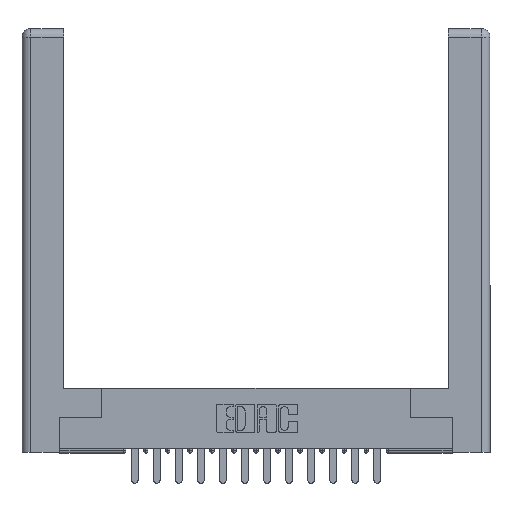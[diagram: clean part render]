
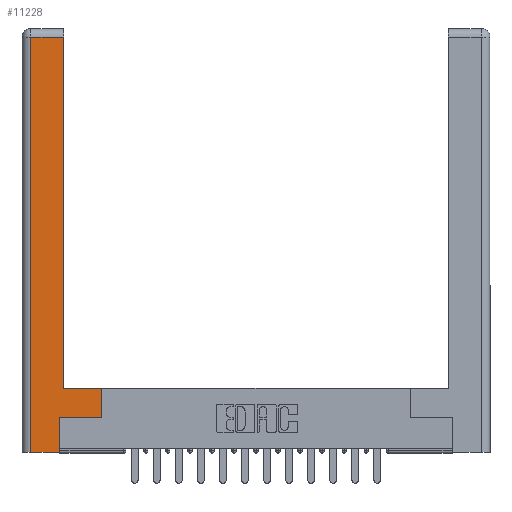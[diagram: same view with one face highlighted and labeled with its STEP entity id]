
A CAD part, top view. The second image highlights one B-rep face of the part: STEP entity #11228.
In plain terms, the highlighted planar face has unit normal (0, 0, 1).
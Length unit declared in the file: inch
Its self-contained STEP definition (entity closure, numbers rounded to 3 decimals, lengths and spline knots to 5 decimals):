
#159 = VECTOR ( 'NONE', #10694, 39.37008 ) ;
#161 = CARTESIAN_POINT ( 'NONE',  ( 0.565, 0.245, 0. ) ) ;
#164 = ORIENTED_EDGE ( 'NONE', *, *, #7320, .T. ) ;
#1499 = EDGE_CURVE ( 'NONE', #12474, #10708, #16077, .T. ) ;
#1503 = EDGE_CURVE ( 'NONE', #18633, #8647, #7940, .T. ) ;
#1504 = DIRECTION ( 'NONE',  ( 1., 0., 0. ) ) ;
#1714 = CARTESIAN_POINT ( 'NONE',  ( 0.295, 3., 0. ) ) ;
#1755 = DIRECTION ( 'NONE',  ( 0., -1., 0. ) ) ;
#2176 = VECTOR ( 'NONE', #12103, 39.37008 ) ;
#2252 = AXIS2_PLACEMENT_3D ( 'NONE', #10477, #3153, #14984 ) ;
#2277 = VECTOR ( 'NONE', #12671, 39.37008 ) ;
#2323 = CARTESIAN_POINT ( 'NONE',  ( 0.295, 2.94, 0. ) ) ;
#2669 = ORIENTED_EDGE ( 'NONE', *, *, #18266, .T. ) ;
#2887 = VECTOR ( 'NONE', #1504, 39.37008 ) ;
#3153 = DIRECTION ( 'NONE',  ( 0., 0., -1. ) ) ;
#3246 = CARTESIAN_POINT ( 'NONE',  ( 0.265, 0.245, 0. ) ) ;
#3468 = EDGE_LOOP ( 'NONE', ( #6511, #2669, #12548, #16633, #18018, #6782, #164, #15457 ) ) ;
#4203 = FACE_OUTER_BOUND ( 'NONE', #3468, .T. ) ;
#4240 = VECTOR ( 'NONE', #1755, 39.37008 ) ;
#5693 = CARTESIAN_POINT ( 'NONE',  ( 0.0615, 2.94, 0. ) ) ;
#6391 = EDGE_CURVE ( 'NONE', #10708, #11615, #10621, .T. ) ;
#6511 = ORIENTED_EDGE ( 'NONE', *, *, #16012, .T. ) ;
#6564 = DIRECTION ( 'NONE',  ( 0., 1., 0. ) ) ;
#6698 = VECTOR ( 'NONE', #16468, 39.37008 ) ;
#6782 = ORIENTED_EDGE ( 'NONE', *, *, #1503, .T. ) ;
#7222 = DIRECTION ( 'NONE',  ( 1., 0., 0. ) ) ;
#7320 = EDGE_CURVE ( 'NONE', #8647, #16659, #12195, .T. ) ;
#7625 = CARTESIAN_POINT ( 'NONE',  ( 0.565, 0.45, 0. ) ) ;
#7712 = VERTEX_POINT ( 'NONE', #18639 ) ;
#7940 = LINE ( 'NONE', #161, #2887 ) ;
#8034 = EDGE_CURVE ( 'NONE', #11615, #18633, #19176, .T. ) ;
#8073 = CARTESIAN_POINT ( 'NONE',  ( 0.565, 0.245, 0. ) ) ;
#8647 = VERTEX_POINT ( 'NONE', #8073 ) ;
#9326 = CARTESIAN_POINT ( 'NONE',  ( 0.295, 0.45, 0. ) ) ;
#10466 = CARTESIAN_POINT ( 'NONE',  ( 0.0615, 2.94, 0. ) ) ;
#10477 = CARTESIAN_POINT ( 'NONE',  ( 0., 0., 0. ) ) ;
#10489 = LINE ( 'NONE', #1714, #2176 ) ;
#10621 = LINE ( 'NONE', #16116, #14840 ) ;
#10694 = DIRECTION ( 'NONE',  ( -1., 0., 0. ) ) ;
#10708 = VERTEX_POINT ( 'NONE', #18716 ) ;
#11228 = ADVANCED_FACE ( 'NONE', ( #4203 ), #12084, .F. ) ;
#11590 = VERTEX_POINT ( 'NONE', #2323 ) ;
#11615 = VERTEX_POINT ( 'NONE', #12589 ) ;
#11921 = LINE ( 'NONE', #9326, #159 ) ;
#12084 = PLANE ( 'NONE',  #2252 ) ;
#12103 = DIRECTION ( 'NONE',  ( 0., 1., 0. ) ) ;
#12195 = LINE ( 'NONE', #18594, #2277 ) ;
#12474 = VERTEX_POINT ( 'NONE', #5693 ) ;
#12548 = ORIENTED_EDGE ( 'NONE', *, *, #1499, .T. ) ;
#12589 = CARTESIAN_POINT ( 'NONE',  ( 0.265, 0., 0. ) ) ;
#12671 = DIRECTION ( 'NONE',  ( 0., 1., 0. ) ) ;
#14129 = LINE ( 'NONE', #10466, #6698 ) ;
#14187 = CARTESIAN_POINT ( 'NONE',  ( 0.265, 0.245, 0. ) ) ;
#14769 = VECTOR ( 'NONE', #6564, 39.37008 ) ;
#14840 = VECTOR ( 'NONE', #7222, 39.37008 ) ;
#14984 = DIRECTION ( 'NONE',  ( -1., 0., 0. ) ) ;
#15039 = EDGE_CURVE ( 'NONE', #16659, #7712, #11921, .T. ) ;
#15457 = ORIENTED_EDGE ( 'NONE', *, *, #15039, .T. ) ;
#16012 = EDGE_CURVE ( 'NONE', #7712, #11590, #10489, .T. ) ;
#16077 = LINE ( 'NONE', #17824, #4240 ) ;
#16116 = CARTESIAN_POINT ( 'NONE',  ( 0.265, 0., 0. ) ) ;
#16468 = DIRECTION ( 'NONE',  ( -1., 0., 0. ) ) ;
#16633 = ORIENTED_EDGE ( 'NONE', *, *, #6391, .T. ) ;
#16659 = VERTEX_POINT ( 'NONE', #7625 ) ;
#17824 = CARTESIAN_POINT ( 'NONE',  ( 0.0615, 0., 0. ) ) ;
#18018 = ORIENTED_EDGE ( 'NONE', *, *, #8034, .T. ) ;
#18266 = EDGE_CURVE ( 'NONE', #11590, #12474, #14129, .T. ) ;
#18594 = CARTESIAN_POINT ( 'NONE',  ( 0.565, 0.45, 0. ) ) ;
#18633 = VERTEX_POINT ( 'NONE', #14187 ) ;
#18639 = CARTESIAN_POINT ( 'NONE',  ( 0.295, 0.45, 0. ) ) ;
#18716 = CARTESIAN_POINT ( 'NONE',  ( 0.0615, 0., 0. ) ) ;
#19176 = LINE ( 'NONE', #3246, #14769 ) ;
